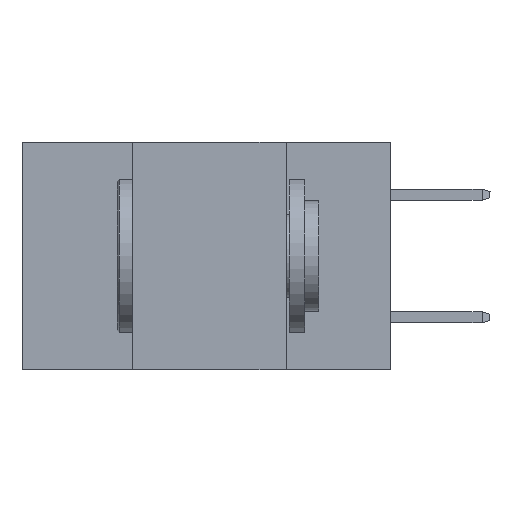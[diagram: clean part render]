
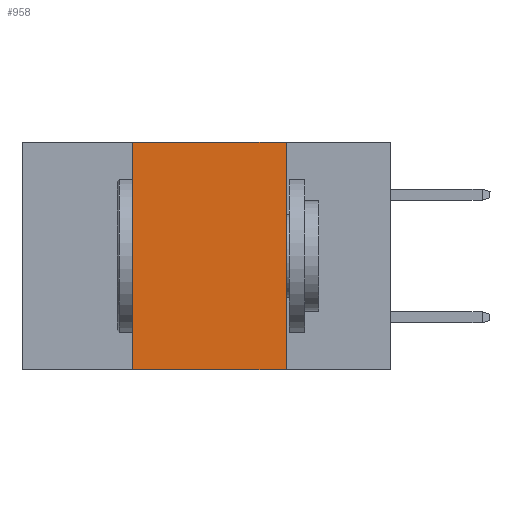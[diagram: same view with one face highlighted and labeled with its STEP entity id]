
A CAD part, left-side view. The second image highlights one B-rep face of the part: STEP entity #958.
In plain terms, the highlighted planar face has unit normal (-1, 0, 0).
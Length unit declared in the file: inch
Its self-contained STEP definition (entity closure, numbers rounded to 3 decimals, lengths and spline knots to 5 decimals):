
#430 = VECTOR ( 'NONE', #9065, 39.37008 ) ;
#524 = CARTESIAN_POINT ( 'NONE',  ( 0., 0.42, -0.37 ) ) ;
#690 = DIRECTION ( 'NONE',  ( 0., 0., -1. ) ) ;
#958 = ADVANCED_FACE ( 'NONE', ( #9530 ), #6052, .F. ) ;
#1403 = DIRECTION ( 'NONE',  ( 1., 0., 0. ) ) ;
#1496 = CARTESIAN_POINT ( 'NONE',  ( 0., 0.6, 0. ) ) ;
#1536 = CARTESIAN_POINT ( 'NONE',  ( 0., 0.17, 0. ) ) ;
#1980 = VERTEX_POINT ( 'NONE', #524 ) ;
#2242 = VERTEX_POINT ( 'NONE', #8063 ) ;
#2360 = CARTESIAN_POINT ( 'NONE',  ( 0., 0.6, -0.37 ) ) ;
#3269 = ORIENTED_EDGE ( 'NONE', *, *, #20006, .T. ) ;
#3713 = DIRECTION ( 'NONE',  ( 0., 0., 1. ) ) ;
#4064 = CARTESIAN_POINT ( 'NONE',  ( 0., 0.17, -0.37 ) ) ;
#4235 = DIRECTION ( 'NONE',  ( 0., 0., -1. ) ) ;
#4266 = VECTOR ( 'NONE', #16481, 39.37008 ) ;
#5617 = VECTOR ( 'NONE', #3713, 39.37008 ) ;
#5701 = EDGE_CURVE ( 'NONE', #2242, #14190, #14723, .T. ) ;
#6052 = PLANE ( 'NONE',  #19387 ) ;
#6534 = EDGE_CURVE ( 'NONE', #1980, #2242, #15479, .T. ) ;
#7002 = ORIENTED_EDGE ( 'NONE', *, *, #16272, .F. ) ;
#7192 = CARTESIAN_POINT ( 'NONE',  ( 0., 0.6, 0. ) ) ;
#8063 = CARTESIAN_POINT ( 'NONE',  ( 0., 0.42, 0. ) ) ;
#9065 = DIRECTION ( 'NONE',  ( 0., -1., 0. ) ) ;
#9530 = FACE_OUTER_BOUND ( 'NONE', #13865, .T. ) ;
#9843 = CARTESIAN_POINT ( 'NONE',  ( 0., 0.17, 0. ) ) ;
#11964 = LINE ( 'NONE', #9843, #20490 ) ;
#13865 = EDGE_LOOP ( 'NONE', ( #7002, #16213, #20764, #3269 ) ) ;
#14190 = VERTEX_POINT ( 'NONE', #1536 ) ;
#14723 = LINE ( 'NONE', #7192, #430 ) ;
#15479 = LINE ( 'NONE', #16009, #5617 ) ;
#16009 = CARTESIAN_POINT ( 'NONE',  ( 0., 0.42, 0. ) ) ;
#16213 = ORIENTED_EDGE ( 'NONE', *, *, #5701, .F. ) ;
#16272 = EDGE_CURVE ( 'NONE', #14190, #19948, #11964, .T. ) ;
#16481 = DIRECTION ( 'NONE',  ( 0., -1., 0. ) ) ;
#18213 = LINE ( 'NONE', #2360, #4266 ) ;
#19387 = AXIS2_PLACEMENT_3D ( 'NONE', #1496, #1403, #4235 ) ;
#19948 = VERTEX_POINT ( 'NONE', #4064 ) ;
#20006 = EDGE_CURVE ( 'NONE', #1980, #19948, #18213, .T. ) ;
#20490 = VECTOR ( 'NONE', #690, 39.37008 ) ;
#20764 = ORIENTED_EDGE ( 'NONE', *, *, #6534, .F. ) ;
